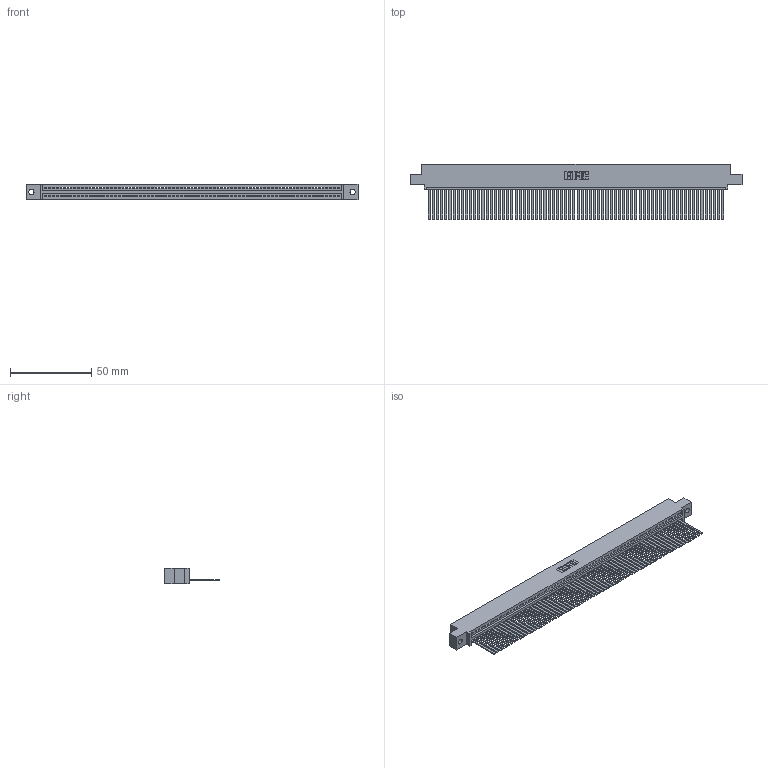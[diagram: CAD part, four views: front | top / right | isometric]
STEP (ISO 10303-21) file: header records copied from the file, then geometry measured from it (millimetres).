
FILE_DESCRIPTION (( 'STEP AP203' ), '1' );
FILE_NAME ('395-072-544-402.STEP', '2018-11-27T14:37:35', ( '' ), ( '' ), 'SwSTEP 2.0', 'SolidWorks 2016', '' );
FILE_SCHEMA (( 'CONFIG_CONTROL_DESIGN' ));
Length unit declared in the file: inch
Products named in the file (3): 345-292-001_345-293-144; 345 Part_0.110 Offset - 0.128 Dia; 395-072-544-402
Assembly tree (73 placements, depth 2):
  395-072-544-402
    345 Part_0.110 Offset - 0.128 Dia
    345-292-001_345-293-144  x72
Bounding box: 204.09 x 33.96 x 9.4 mm (x, y, z)
Volume: 20354.1 mm3; surface area: 29770.2 mm2
Topology: 73 solids, 73 shells, 3874 faces, 11729 edges, 7722 vertices
Faces by surface type: plane 2676, cylinder 1198
Entity records: 50101 total; most frequent: ORIENTED_EDGE 8690, CARTESIAN_POINT 8684, DIRECTION 7537, EDGE_CURVE 4345, VECTOR 3929, LINE 3929, VERTEX_POINT 2894, AXIS2_PLACEMENT_3D 1804
